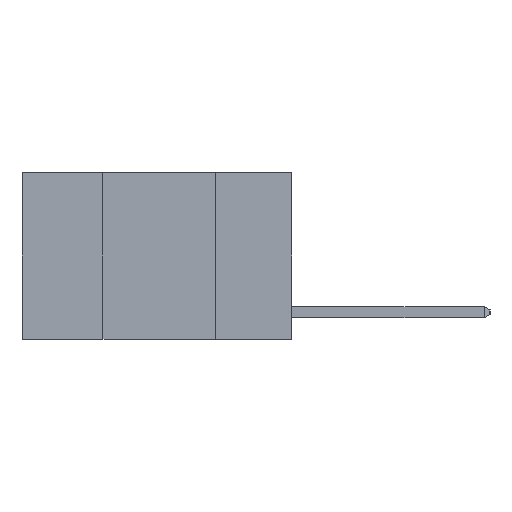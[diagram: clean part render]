
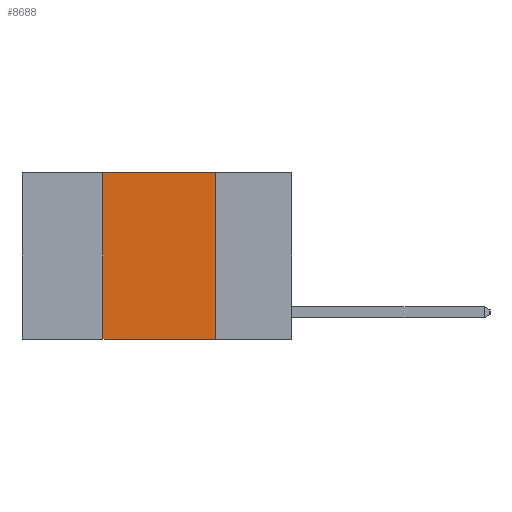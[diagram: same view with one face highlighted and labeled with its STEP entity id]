
A CAD part, left-side view. The second image highlights one B-rep face of the part: STEP entity #8688.
In plain terms, the highlighted planar face has unit normal (-1, 0, 0).
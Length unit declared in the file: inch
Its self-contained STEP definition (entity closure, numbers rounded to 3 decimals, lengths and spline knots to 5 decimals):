
#94 = CARTESIAN_POINT ( 'NONE',  ( 0., 0.42, 0. ) ) ;
#201 = CARTESIAN_POINT ( 'NONE',  ( 0., 0.17, 0. ) ) ;
#544 = VERTEX_POINT ( 'NONE', #201 ) ;
#619 = VECTOR ( 'NONE', #8189, 39.37008 ) ;
#1475 = VERTEX_POINT ( 'NONE', #4338 ) ;
#2167 = FACE_OUTER_BOUND ( 'NONE', #4902, .T. ) ;
#2663 = PLANE ( 'NONE',  #9619 ) ;
#2716 = CARTESIAN_POINT ( 'NONE',  ( 0., 0.6, -0.37 ) ) ;
#3830 = CARTESIAN_POINT ( 'NONE',  ( 0., 0.17, 0. ) ) ;
#3909 = EDGE_CURVE ( 'NONE', #1475, #4004, #7534, .T. ) ;
#4004 = VERTEX_POINT ( 'NONE', #94 ) ;
#4088 = DIRECTION ( 'NONE',  ( 0., 0., 1. ) ) ;
#4198 = LINE ( 'NONE', #2716, #8178 ) ;
#4338 = CARTESIAN_POINT ( 'NONE',  ( 0., 0.42, -0.37 ) ) ;
#4373 = EDGE_CURVE ( 'NONE', #4004, #544, #9207, .T. ) ;
#4400 = DIRECTION ( 'NONE',  ( 1., 0., 0. ) ) ;
#4445 = EDGE_CURVE ( 'NONE', #1475, #9303, #4198, .T. ) ;
#4902 = EDGE_LOOP ( 'NONE', ( #8093, #9833, #9240, #9963 ) ) ;
#5129 = DIRECTION ( 'NONE',  ( 0., -1., 0. ) ) ;
#5942 = VECTOR ( 'NONE', #4088, 39.37008 ) ;
#6879 = CARTESIAN_POINT ( 'NONE',  ( 0., 0.17, -0.37 ) ) ;
#7289 = EDGE_CURVE ( 'NONE', #544, #9303, #8266, .T. ) ;
#7358 = CARTESIAN_POINT ( 'NONE',  ( 0., 0.6, 0. ) ) ;
#7534 = LINE ( 'NONE', #9659, #5942 ) ;
#8093 = ORIENTED_EDGE ( 'NONE', *, *, #7289, .F. ) ;
#8178 = VECTOR ( 'NONE', #5129, 39.37008 ) ;
#8189 = DIRECTION ( 'NONE',  ( 0., -1., 0. ) ) ;
#8266 = LINE ( 'NONE', #3830, #10346 ) ;
#8612 = DIRECTION ( 'NONE',  ( 0., 0., -1. ) ) ;
#8688 = ADVANCED_FACE ( 'NONE', ( #2167 ), #2663, .F. ) ;
#9203 = CARTESIAN_POINT ( 'NONE',  ( 0., 0.6, 0. ) ) ;
#9207 = LINE ( 'NONE', #7358, #619 ) ;
#9240 = ORIENTED_EDGE ( 'NONE', *, *, #3909, .F. ) ;
#9303 = VERTEX_POINT ( 'NONE', #6879 ) ;
#9619 = AXIS2_PLACEMENT_3D ( 'NONE', #9203, #4400, #9969 ) ;
#9659 = CARTESIAN_POINT ( 'NONE',  ( 0., 0.42, 0. ) ) ;
#9833 = ORIENTED_EDGE ( 'NONE', *, *, #4373, .F. ) ;
#9963 = ORIENTED_EDGE ( 'NONE', *, *, #4445, .T. ) ;
#9969 = DIRECTION ( 'NONE',  ( 0., 0., -1. ) ) ;
#10346 = VECTOR ( 'NONE', #8612, 39.37008 ) ;
